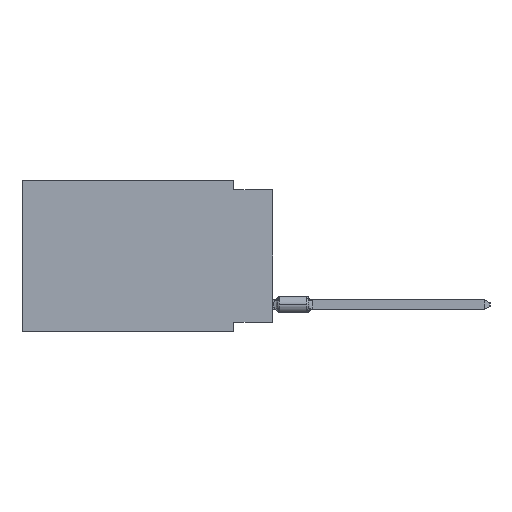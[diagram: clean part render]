
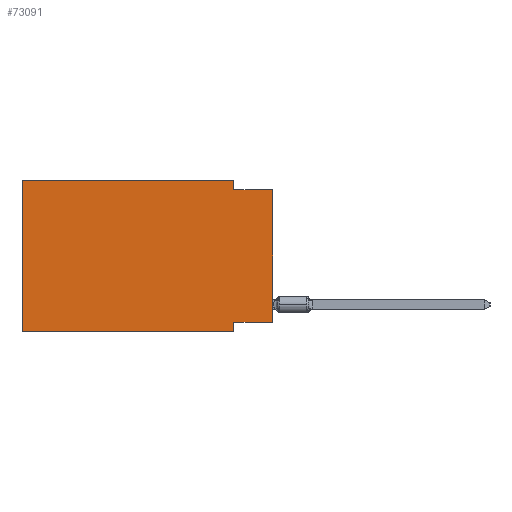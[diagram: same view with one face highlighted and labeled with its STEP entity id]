
A CAD part, left-side view. The second image highlights one B-rep face of the part: STEP entity #73091.
In plain terms, the highlighted planar face has unit normal (-1, 0, 0).
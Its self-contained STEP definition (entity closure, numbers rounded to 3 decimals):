
#812 = VECTOR ( 'NONE', #33164, 1000. ) ;
#1351 = LINE ( 'NONE', #26881, #25522 ) ;
#1691 = LINE ( 'NONE', #39945, #812 ) ;
#1704 = DIRECTION ( 'NONE',  ( 0., 1., 0. ) ) ;
#3237 = VECTOR ( 'NONE', #29441, 1000. ) ;
#5121 = CARTESIAN_POINT ( 'NONE',  ( 0., 2.54, 0. ) ) ;
#5948 = ORIENTED_EDGE ( 'NONE', *, *, #30775, .F. ) ;
#6827 = VERTEX_POINT ( 'NONE', #38724 ) ;
#9779 = DIRECTION ( 'NONE',  ( 1., 0., 0. ) ) ;
#12711 = CARTESIAN_POINT ( 'NONE',  ( 0., 2.54, -9.906 ) ) ;
#17518 = EDGE_CURVE ( 'NONE', #43256, #68104, #59696, .T. ) ;
#20970 = AXIS2_PLACEMENT_3D ( 'NONE', #76045, #9779, #29765 ) ;
#22559 = PLANE ( 'NONE',  #20970 ) ;
#23838 = FACE_OUTER_BOUND ( 'NONE', #79807, .T. ) ;
#25522 = VECTOR ( 'NONE', #83810, 1000. ) ;
#26881 = CARTESIAN_POINT ( 'NONE',  ( 0., 16.383, 0. ) ) ;
#28395 = ORIENTED_EDGE ( 'NONE', *, *, #71122, .F. ) ;
#29441 = DIRECTION ( 'NONE',  ( 0., 0., -1. ) ) ;
#29765 = DIRECTION ( 'NONE',  ( 0., 0., -1. ) ) ;
#30035 = VECTOR ( 'NONE', #72109, 1000. ) ;
#30775 = EDGE_CURVE ( 'NONE', #43256, #6827, #65023, .T. ) ;
#31862 = DIRECTION ( 'NONE',  ( 0., 0., -1. ) ) ;
#32105 = CARTESIAN_POINT ( 'NONE',  ( 0., 0., -0.635 ) ) ;
#33164 = DIRECTION ( 'NONE',  ( 0., 0., 1. ) ) ;
#33179 = CARTESIAN_POINT ( 'NONE',  ( 0., 0., -9.271 ) ) ;
#36382 = ORIENTED_EDGE ( 'NONE', *, *, #65846, .F. ) ;
#36972 = VERTEX_POINT ( 'NONE', #49229 ) ;
#37092 = EDGE_CURVE ( 'NONE', #36972, #64856, #1351, .T. ) ;
#38724 = CARTESIAN_POINT ( 'NONE',  ( 0., 2.54, -9.271 ) ) ;
#39878 = LINE ( 'NONE', #12711, #75187 ) ;
#39945 = CARTESIAN_POINT ( 'NONE',  ( 0., 16.383, 0. ) ) ;
#41464 = CARTESIAN_POINT ( 'NONE',  ( 0., 2.54, -0.635 ) ) ;
#43256 = VERTEX_POINT ( 'NONE', #80896 ) ;
#44457 = ORIENTED_EDGE ( 'NONE', *, *, #58845, .F. ) ;
#44742 = EDGE_CURVE ( 'NONE', #53586, #59002, #64917, .T. ) ;
#45252 = LINE ( 'NONE', #32105, #67767 ) ;
#49229 = CARTESIAN_POINT ( 'NONE',  ( 0., 16.383, 0. ) ) ;
#49371 = LINE ( 'NONE', #54907, #3237 ) ;
#49896 = EDGE_CURVE ( 'NONE', #53586, #36972, #1691, .T. ) ;
#51468 = CARTESIAN_POINT ( 'NONE',  ( 0., 2.54, -9.906 ) ) ;
#52164 = CARTESIAN_POINT ( 'NONE',  ( 0., 16.383, -9.906 ) ) ;
#53586 = VERTEX_POINT ( 'NONE', #83249 ) ;
#54907 = CARTESIAN_POINT ( 'NONE',  ( 0., 2.54, 0. ) ) ;
#56544 = ORIENTED_EDGE ( 'NONE', *, *, #44742, .T. ) ;
#57998 = DIRECTION ( 'NONE',  ( 0., -1., 0. ) ) ;
#58691 = VECTOR ( 'NONE', #1704, 1000. ) ;
#58845 = EDGE_CURVE ( 'NONE', #64856, #61003, #49371, .T. ) ;
#59002 = VERTEX_POINT ( 'NONE', #51468 ) ;
#59696 = LINE ( 'NONE', #66485, #68965 ) ;
#61003 = VERTEX_POINT ( 'NONE', #41464 ) ;
#64856 = VERTEX_POINT ( 'NONE', #5121 ) ;
#64917 = LINE ( 'NONE', #52164, #30035 ) ;
#65023 = LINE ( 'NONE', #33179, #58691 ) ;
#65846 = EDGE_CURVE ( 'NONE', #61003, #68104, #45252, .T. ) ;
#66485 = CARTESIAN_POINT ( 'NONE',  ( 0., 0., 0. ) ) ;
#67767 = VECTOR ( 'NONE', #57998, 1000. ) ;
#68104 = VERTEX_POINT ( 'NONE', #76411 ) ;
#68965 = VECTOR ( 'NONE', #80048, 1000. ) ;
#69344 = ORIENTED_EDGE ( 'NONE', *, *, #49896, .F. ) ;
#70919 = ORIENTED_EDGE ( 'NONE', *, *, #17518, .T. ) ;
#71122 = EDGE_CURVE ( 'NONE', #6827, #59002, #39878, .T. ) ;
#72109 = DIRECTION ( 'NONE',  ( 0., -1., 0. ) ) ;
#73091 = ADVANCED_FACE ( 'NONE', ( #23838 ), #22559, .F. ) ;
#75187 = VECTOR ( 'NONE', #31862, 1000. ) ;
#76045 = CARTESIAN_POINT ( 'NONE',  ( 0., 16.383, 0. ) ) ;
#76411 = CARTESIAN_POINT ( 'NONE',  ( 0., 0., -0.635 ) ) ;
#79807 = EDGE_LOOP ( 'NONE', ( #70919, #36382, #44457, #83256, #69344, #56544, #28395, #5948 ) ) ;
#80048 = DIRECTION ( 'NONE',  ( 0., 0., 1. ) ) ;
#80896 = CARTESIAN_POINT ( 'NONE',  ( 0., 0., -9.271 ) ) ;
#83249 = CARTESIAN_POINT ( 'NONE',  ( 0., 16.383, -9.906 ) ) ;
#83256 = ORIENTED_EDGE ( 'NONE', *, *, #37092, .F. ) ;
#83810 = DIRECTION ( 'NONE',  ( 0., -1., 0. ) ) ;
